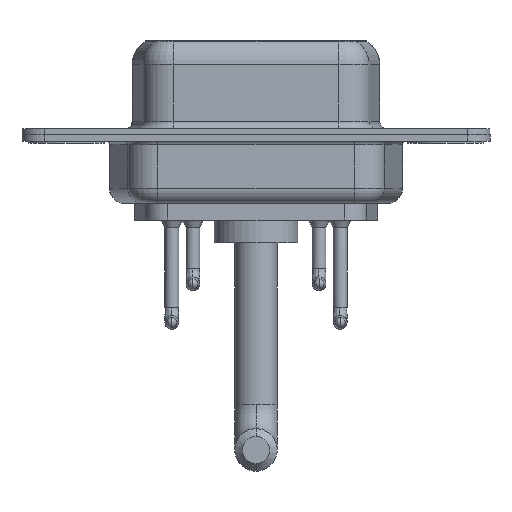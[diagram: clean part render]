
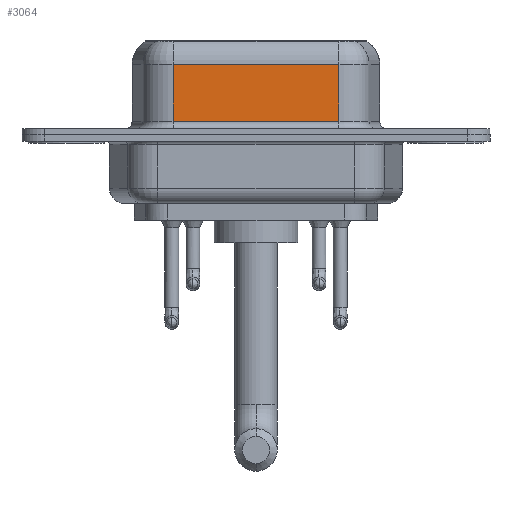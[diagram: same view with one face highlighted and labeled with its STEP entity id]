
A CAD part, front view. The second image highlights one B-rep face of the part: STEP entity #3064.
In plain terms, the highlighted planar face has unit normal (0, -1, 0).
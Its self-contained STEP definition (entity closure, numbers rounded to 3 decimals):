
#86 = ORIENTED_EDGE ( 'NONE', *, *, #2377, .T. ) ;
#301 = EDGE_CURVE ( 'NONE', #1681, #11593, #3565, .T. ) ;
#624 = CARTESIAN_POINT ( 'NONE',  ( 17.962, -3.95, 4.65 ) ) ;
#814 = CARTESIAN_POINT ( 'NONE',  ( 7.038, -3.95, 6.4 ) ) ;
#952 = DIRECTION ( 'NONE',  ( -1., 0., 0. ) ) ;
#1024 = LINE ( 'NONE', #11079, #10257 ) ;
#1150 = CARTESIAN_POINT ( 'NONE',  ( 17.962, -3.95, 6.4 ) ) ;
#1247 = LINE ( 'NONE', #12256, #13591 ) ;
#1681 = VERTEX_POINT ( 'NONE', #624 ) ;
#2107 = EDGE_CURVE ( 'NONE', #10810, #13358, #13288, .T. ) ;
#2377 = EDGE_CURVE ( 'NONE', #1681, #10810, #1024, .T. ) ;
#3064 = ADVANCED_FACE ( 'NONE', ( #5143 ), #4988, .F. ) ;
#3259 = ORIENTED_EDGE ( 'NONE', *, *, #2107, .T. ) ;
#3565 = LINE ( 'NONE', #1150, #11225 ) ;
#4923 = CARTESIAN_POINT ( 'NONE',  ( 17.962, -3.95, 6.4 ) ) ;
#4988 = PLANE ( 'NONE',  #6940 ) ;
#5143 = FACE_OUTER_BOUND ( 'NONE', #8755, .T. ) ;
#5623 = DIRECTION ( 'NONE',  ( 0., 0., -1. ) ) ;
#6127 = EDGE_CURVE ( 'NONE', #13358, #11593, #1247, .T. ) ;
#6940 = AXIS2_PLACEMENT_3D ( 'NONE', #4923, #9496, #9714 ) ;
#7619 = ORIENTED_EDGE ( 'NONE', *, *, #6127, .T. ) ;
#7785 = DIRECTION ( 'NONE',  ( 1., 0., 0. ) ) ;
#8749 = DIRECTION ( 'NONE',  ( 0., 0., -1. ) ) ;
#8755 = EDGE_LOOP ( 'NONE', ( #14521, #86, #3259, #7619 ) ) ;
#9496 = DIRECTION ( 'NONE',  ( 0., 1., 0. ) ) ;
#9714 = DIRECTION ( 'NONE',  ( -1., 0., 0. ) ) ;
#10257 = VECTOR ( 'NONE', #952, 1000. ) ;
#10810 = VERTEX_POINT ( 'NONE', #13431 ) ;
#11079 = CARTESIAN_POINT ( 'NONE',  ( 17.962, -3.95, 4.65 ) ) ;
#11225 = VECTOR ( 'NONE', #5623, 1000. ) ;
#11593 = VERTEX_POINT ( 'NONE', #14320 ) ;
#12256 = CARTESIAN_POINT ( 'NONE',  ( 17.962, -3.95, 0.9 ) ) ;
#13014 = CARTESIAN_POINT ( 'NONE',  ( 7.038, -3.95, 0.9 ) ) ;
#13273 = VECTOR ( 'NONE', #8749, 1000. ) ;
#13288 = LINE ( 'NONE', #814, #13273 ) ;
#13358 = VERTEX_POINT ( 'NONE', #13014 ) ;
#13431 = CARTESIAN_POINT ( 'NONE',  ( 7.038, -3.95, 4.65 ) ) ;
#13591 = VECTOR ( 'NONE', #7785, 1000. ) ;
#14320 = CARTESIAN_POINT ( 'NONE',  ( 17.962, -3.95, 0.9 ) ) ;
#14521 = ORIENTED_EDGE ( 'NONE', *, *, #301, .F. ) ;
